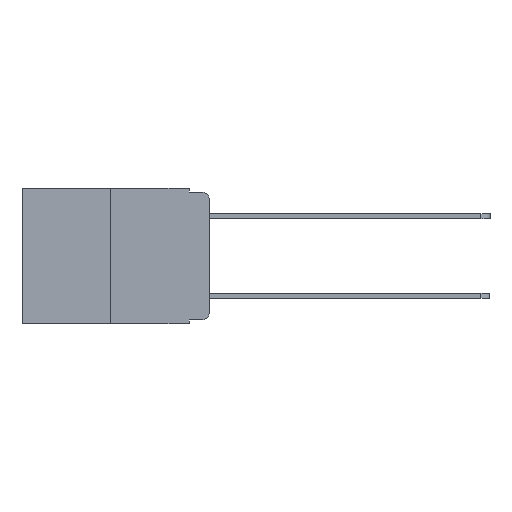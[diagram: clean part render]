
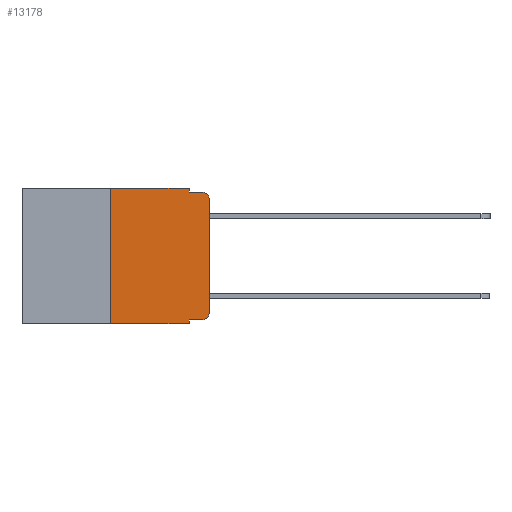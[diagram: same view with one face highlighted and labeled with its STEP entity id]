
A CAD part, left-side view. The second image highlights one B-rep face of the part: STEP entity #13178.
In plain terms, the highlighted planar face has unit normal (-1, 0, 0).
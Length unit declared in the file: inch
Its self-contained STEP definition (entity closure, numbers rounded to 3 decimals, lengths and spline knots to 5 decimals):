
#406 = ORIENTED_EDGE ( 'NONE', *, *, #10493, .T. ) ;
#502 = CARTESIAN_POINT ( 'NONE',  ( 0., 0.051, 0. ) ) ;
#504 = DIRECTION ( 'NONE',  ( 0., -1., 0. ) ) ;
#566 = CARTESIAN_POINT ( 'NONE',  ( 0., 0.051, 0. ) ) ;
#859 = CARTESIAN_POINT ( 'NONE',  ( 0., 0.473, -0.343 ) ) ;
#1015 = CARTESIAN_POINT ( 'NONE',  ( 0., 0.25, 0. ) ) ;
#1136 = ORIENTED_EDGE ( 'NONE', *, *, #8982, .F. ) ;
#1397 = LINE ( 'NONE', #20782, #14434 ) ;
#1476 = VERTEX_POINT ( 'NONE', #9403 ) ;
#1513 = DIRECTION ( 'NONE',  ( 0., 0., 1. ) ) ;
#1541 = VECTOR ( 'NONE', #6048, 39.37008 ) ;
#1833 = EDGE_CURVE ( 'NONE', #21443, #13643, #7575, .T. ) ;
#2109 = DIRECTION ( 'NONE',  ( -1., 0., 0. ) ) ;
#2213 = EDGE_CURVE ( 'NONE', #12710, #1476, #14162, .T. ) ;
#2330 = CARTESIAN_POINT ( 'NONE',  ( 0., 0.473, 0. ) ) ;
#2698 = VECTOR ( 'NONE', #1513, 39.37008 ) ;
#2763 = CARTESIAN_POINT ( 'NONE',  ( 0., 0.051, 0. ) ) ;
#2810 = CARTESIAN_POINT ( 'NONE',  ( 0., 0.25, -0.343 ) ) ;
#3225 = LINE ( 'NONE', #20036, #2698 ) ;
#3957 = VERTEX_POINT ( 'NONE', #6140 ) ;
#4003 = VERTEX_POINT ( 'NONE', #8964 ) ;
#4080 = ORIENTED_EDGE ( 'NONE', *, *, #2213, .F. ) ;
#4453 = DIRECTION ( 'NONE',  ( 0., 0., -1. ) ) ;
#5118 = ORIENTED_EDGE ( 'NONE', *, *, #6441, .F. ) ;
#5443 = AXIS2_PLACEMENT_3D ( 'NONE', #7282, #9136, #20932 ) ;
#5560 = DIRECTION ( 'NONE',  ( 0., -1., 0. ) ) ;
#5721 = EDGE_CURVE ( 'NONE', #15572, #21443, #12991, .T. ) ;
#5758 = DIRECTION ( 'NONE',  ( 0., 0., -1. ) ) ;
#6048 = DIRECTION ( 'NONE',  ( 0., -1., 0. ) ) ;
#6140 = CARTESIAN_POINT ( 'NONE',  ( 0., 0.051, -0.01 ) ) ;
#6441 = EDGE_CURVE ( 'NONE', #1476, #16128, #8466, .T. ) ;
#6777 = DIRECTION ( 'NONE',  ( -1., 0., 0. ) ) ;
#6802 = CARTESIAN_POINT ( 'NONE',  ( 0., 0.02, -0.03 ) ) ;
#7282 = CARTESIAN_POINT ( 'NONE',  ( 0., 0.473, 0. ) ) ;
#7481 = ORIENTED_EDGE ( 'NONE', *, *, #5721, .T. ) ;
#7575 = CIRCLE ( 'NONE', #12267, 0.02 ) ;
#7951 = VECTOR ( 'NONE', #504, 39.37008 ) ;
#8301 = DIRECTION ( 'NONE',  ( 0., 0., -1. ) ) ;
#8466 = LINE ( 'NONE', #2330, #7951 ) ;
#8666 = EDGE_CURVE ( 'NONE', #4003, #9881, #16314, .T. ) ;
#8964 = CARTESIAN_POINT ( 'NONE',  ( 0., 0., -0.03 ) ) ;
#8982 = EDGE_CURVE ( 'NONE', #3957, #9881, #1397, .T. ) ;
#9136 = DIRECTION ( 'NONE',  ( 1., 0., 0. ) ) ;
#9403 = CARTESIAN_POINT ( 'NONE',  ( 0., 0.25, 0. ) ) ;
#9642 = EDGE_LOOP ( 'NONE', ( #406, #16069, #1136, #17367, #5118, #4080, #17278, #15562, #7481, #10211 ) ) ;
#9661 = EDGE_CURVE ( 'NONE', #15572, #17621, #19685, .T. ) ;
#9881 = VERTEX_POINT ( 'NONE', #11448 ) ;
#10104 = FACE_OUTER_BOUND ( 'NONE', #9642, .T. ) ;
#10211 = ORIENTED_EDGE ( 'NONE', *, *, #1833, .T. ) ;
#10493 = EDGE_CURVE ( 'NONE', #13643, #4003, #3225, .T. ) ;
#10548 = CARTESIAN_POINT ( 'NONE',  ( 0., 0.02, -0.333 ) ) ;
#10833 = DIRECTION ( 'NONE',  ( 0., 0., -1. ) ) ;
#11448 = CARTESIAN_POINT ( 'NONE',  ( 0., 0.02, -0.01 ) ) ;
#12267 = AXIS2_PLACEMENT_3D ( 'NONE', #15433, #2109, #8301 ) ;
#12397 = CARTESIAN_POINT ( 'NONE',  ( 0., 0.051, -0.333 ) ) ;
#12710 = VERTEX_POINT ( 'NONE', #2810 ) ;
#12743 = LINE ( 'NONE', #2763, #21179 ) ;
#12991 = LINE ( 'NONE', #15620, #16963 ) ;
#13178 = ADVANCED_FACE ( 'NONE', ( #10104 ), #19241, .F. ) ;
#13627 = VECTOR ( 'NONE', #20276, 39.37008 ) ;
#13643 = VERTEX_POINT ( 'NONE', #15457 ) ;
#13933 = EDGE_CURVE ( 'NONE', #16128, #3957, #12743, .T. ) ;
#14162 = LINE ( 'NONE', #1015, #13627 ) ;
#14434 = VECTOR ( 'NONE', #5560, 39.37008 ) ;
#15196 = VECTOR ( 'NONE', #5758, 39.37008 ) ;
#15433 = CARTESIAN_POINT ( 'NONE',  ( 0., 0.02, -0.313 ) ) ;
#15457 = CARTESIAN_POINT ( 'NONE',  ( 0., 0., -0.313 ) ) ;
#15562 = ORIENTED_EDGE ( 'NONE', *, *, #9661, .F. ) ;
#15572 = VERTEX_POINT ( 'NONE', #12397 ) ;
#15620 = CARTESIAN_POINT ( 'NONE',  ( 0., 0.051, -0.333 ) ) ;
#15992 = AXIS2_PLACEMENT_3D ( 'NONE', #6802, #6777, #10833 ) ;
#16069 = ORIENTED_EDGE ( 'NONE', *, *, #8666, .T. ) ;
#16128 = VERTEX_POINT ( 'NONE', #502 ) ;
#16314 = CIRCLE ( 'NONE', #15992, 0.02 ) ;
#16963 = VECTOR ( 'NONE', #20259, 39.37008 ) ;
#17278 = ORIENTED_EDGE ( 'NONE', *, *, #21139, .T. ) ;
#17367 = ORIENTED_EDGE ( 'NONE', *, *, #13933, .F. ) ;
#17621 = VERTEX_POINT ( 'NONE', #19038 ) ;
#19038 = CARTESIAN_POINT ( 'NONE',  ( 0., 0.051, -0.343 ) ) ;
#19077 = LINE ( 'NONE', #859, #1541 ) ;
#19241 = PLANE ( 'NONE',  #5443 ) ;
#19685 = LINE ( 'NONE', #566, #15196 ) ;
#20036 = CARTESIAN_POINT ( 'NONE',  ( 0., 0., 0. ) ) ;
#20259 = DIRECTION ( 'NONE',  ( 0., -1., 0. ) ) ;
#20276 = DIRECTION ( 'NONE',  ( 0., 0., 1. ) ) ;
#20782 = CARTESIAN_POINT ( 'NONE',  ( 0., 0.051, -0.01 ) ) ;
#20932 = DIRECTION ( 'NONE',  ( 0., 0., -1. ) ) ;
#21139 = EDGE_CURVE ( 'NONE', #12710, #17621, #19077, .T. ) ;
#21179 = VECTOR ( 'NONE', #4453, 39.37008 ) ;
#21443 = VERTEX_POINT ( 'NONE', #10548 ) ;
